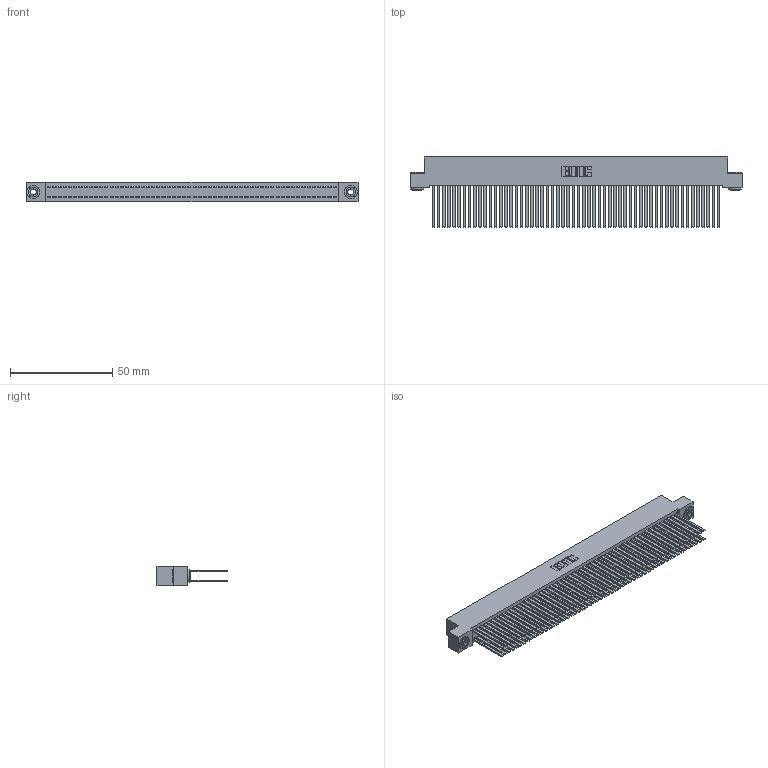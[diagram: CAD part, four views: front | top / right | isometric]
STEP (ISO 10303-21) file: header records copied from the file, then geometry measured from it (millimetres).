
FILE_DESCRIPTION (( 'STEP AP203' ), '1' );
FILE_NAME ('392-112-544-203.STEP', '2019-10-10T00:31:03', ( '' ), ( '' ), 'SwSTEP 2.0', 'SolidWorks 2016', '' );
FILE_SCHEMA (( 'CONFIG_CONTROL_DESIGN' ));
Length unit declared in the file: inch
Products named in the file (4): 392-112-544-203; 342 Part_.156 TH; 345-292-001_345-293-144; 342-250-002_345-250-002-102
Assembly tree (115 placements, depth 2):
  392-112-544-203
    342 Part_.156 TH
    345-292-001_345-293-144  x112
    342-250-002_345-250-002-102  x2
Bounding box: 162.56 x 34.3 x 9.4 mm (x, y, z)
Volume: 16265.1 mm3; surface area: 31382.6 mm2
Topology: 115 solids, 115 shells, 5300 faces, 15719 edges, 10326 vertices
Faces by surface type: plane 3660, cylinder 1632, cone 8
Entity records: 34550 total; most frequent: CARTESIAN_POINT 5681, ORIENTED_EDGE 5610, DIRECTION 4859, EDGE_CURVE 2805, LINE 2657, VECTOR 2657, VERTEX_POINT 1866, AXIS2_PLACEMENT_3D 1101
